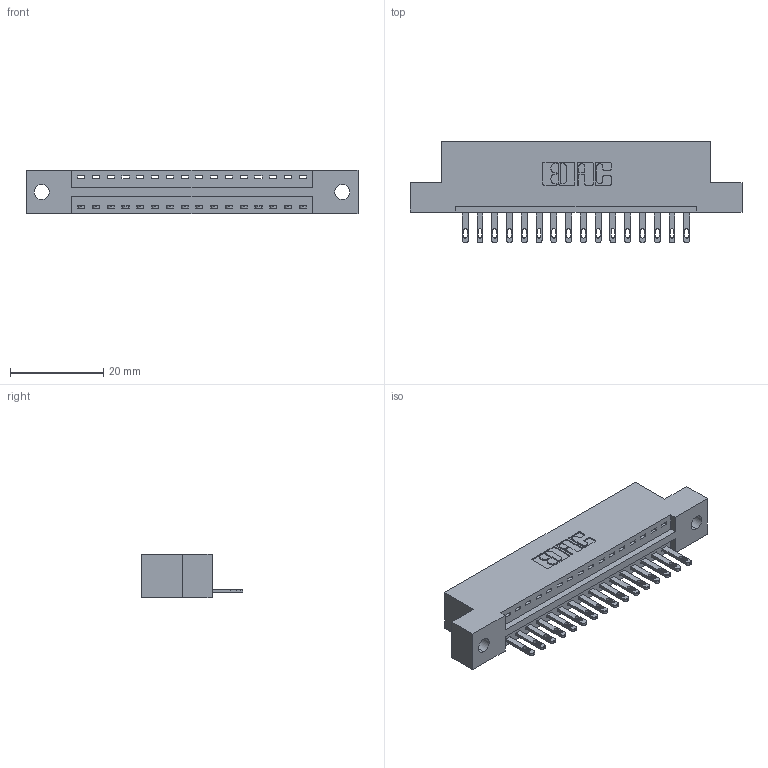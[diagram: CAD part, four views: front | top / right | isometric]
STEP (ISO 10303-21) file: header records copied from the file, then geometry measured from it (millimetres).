
FILE_DESCRIPTION (( 'STEP AP203' ), '1' );
FILE_NAME ('346-016-500-102.STEP', '2022-05-05T09:17:02', ( '' ), ( '' ), 'SwSTEP 2.0', 'SolidWorks 2020', '' );
FILE_SCHEMA (( 'CONFIG_CONTROL_DESIGN' ));
Length unit declared in the file: inch
Products named in the file (3): 345-292-001_345-293-100; 346 Part_Flush Mounting Lugs - 0.128 Dia; 346-016-500-102
Assembly tree (17 placements, depth 2):
  346-016-500-102
    346 Part_Flush Mounting Lugs - 0.128 Dia
    345-292-001_345-293-100  x16
Bounding box: 71.37 x 21.84 x 9.4 mm (x, y, z)
Volume: 6626.2 mm3; surface area: 7767.3 mm2
Topology: 17 solids, 17 shells, 986 faces, 3017 edges, 2010 vertices
Faces by surface type: plane 620, cylinder 366
Entity records: 13363 total; most frequent: CARTESIAN_POINT 2304, ORIENTED_EDGE 2254, DIRECTION 2067, EDGE_CURVE 1127, VECTOR 927, LINE 927, VERTEX_POINT 750, AXIS2_PLACEMENT_3D 570
